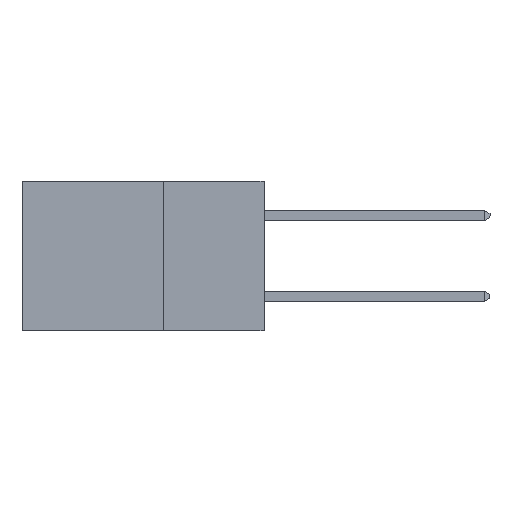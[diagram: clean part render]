
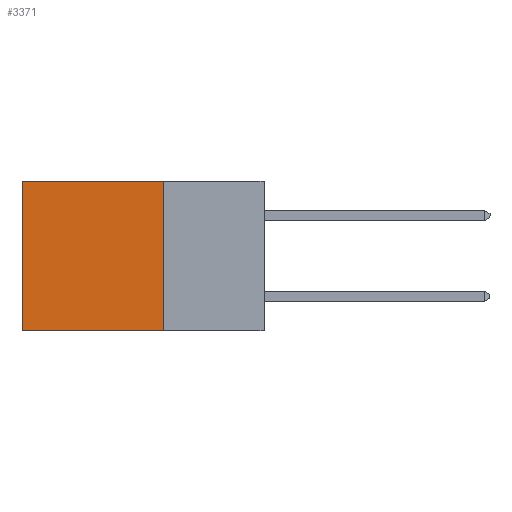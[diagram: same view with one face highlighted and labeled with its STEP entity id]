
A CAD part, left-side view. The second image highlights one B-rep face of the part: STEP entity #3371.
In plain terms, the highlighted planar face has unit normal (-1, 0, 0).
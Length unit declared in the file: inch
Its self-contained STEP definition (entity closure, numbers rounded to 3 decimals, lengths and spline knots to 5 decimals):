
#221 = EDGE_LOOP ( 'NONE', ( #1080, #1675, #1879, #1989 ) ) ;
#222 = EDGE_CURVE ( 'NONE', #11621, #10292, #1241, .T. ) ;
#354 = CARTESIAN_POINT ( 'NONE',  ( 0.298, 0.25, 0. ) ) ;
#417 = LINE ( 'NONE', #4341, #7969 ) ;
#936 = DIRECTION ( 'NONE',  ( 0., 0., -1. ) ) ;
#943 = VECTOR ( 'NONE', #1759, 39.37008 ) ;
#1080 = ORIENTED_EDGE ( 'NONE', *, *, #222, .T. ) ;
#1241 = LINE ( 'NONE', #4678, #943 ) ;
#1675 = ORIENTED_EDGE ( 'NONE', *, *, #11121, .F. ) ;
#1759 = DIRECTION ( 'NONE',  ( 0., 0., -1. ) ) ;
#1879 = ORIENTED_EDGE ( 'NONE', *, *, #4227, .F. ) ;
#1989 = ORIENTED_EDGE ( 'NONE', *, *, #6055, .T. ) ;
#2547 = PLANE ( 'NONE',  #6937 ) ;
#2744 = VECTOR ( 'NONE', #936, 39.37008 ) ;
#3371 = ADVANCED_FACE ( 'NONE', ( #6474 ), #2547, .F. ) ;
#4006 = VECTOR ( 'NONE', #8248, 39.37008 ) ;
#4227 = EDGE_CURVE ( 'NONE', #7983, #10076, #5371, .T. ) ;
#4314 = LINE ( 'NONE', #11914, #4006 ) ;
#4341 = CARTESIAN_POINT ( 'NONE',  ( 0.298, 0.25, 0. ) ) ;
#4498 = CARTESIAN_POINT ( 'NONE',  ( 0.298, 0.25, 0. ) ) ;
#4678 = CARTESIAN_POINT ( 'NONE',  ( 0.298, 0.6, 0. ) ) ;
#5371 = LINE ( 'NONE', #8763, #2744 ) ;
#5376 = DIRECTION ( 'NONE',  ( 0., 1., 0. ) ) ;
#5525 = DIRECTION ( 'NONE',  ( 0., 0., -1. ) ) ;
#6055 = EDGE_CURVE ( 'NONE', #7983, #11621, #417, .T. ) ;
#6474 = FACE_OUTER_BOUND ( 'NONE', #221, .T. ) ;
#6937 = AXIS2_PLACEMENT_3D ( 'NONE', #4498, #11167, #5525 ) ;
#7056 = CARTESIAN_POINT ( 'NONE',  ( 0.298, 0.25, -0.37 ) ) ;
#7915 = CARTESIAN_POINT ( 'NONE',  ( 0.298, 0.6, 0. ) ) ;
#7969 = VECTOR ( 'NONE', #5376, 39.37008 ) ;
#7983 = VERTEX_POINT ( 'NONE', #354 ) ;
#8248 = DIRECTION ( 'NONE',  ( 0., 1., 0. ) ) ;
#8763 = CARTESIAN_POINT ( 'NONE',  ( 0.298, 0.25, 0. ) ) ;
#10076 = VERTEX_POINT ( 'NONE', #7056 ) ;
#10292 = VERTEX_POINT ( 'NONE', #11883 ) ;
#11121 = EDGE_CURVE ( 'NONE', #10076, #10292, #4314, .T. ) ;
#11167 = DIRECTION ( 'NONE',  ( 1., 0., 0. ) ) ;
#11621 = VERTEX_POINT ( 'NONE', #7915 ) ;
#11883 = CARTESIAN_POINT ( 'NONE',  ( 0.298, 0.6, -0.37 ) ) ;
#11914 = CARTESIAN_POINT ( 'NONE',  ( 0.298, 0.25, -0.37 ) ) ;
